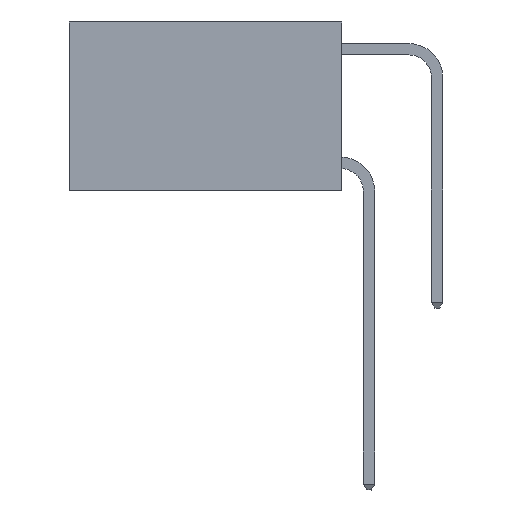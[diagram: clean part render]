
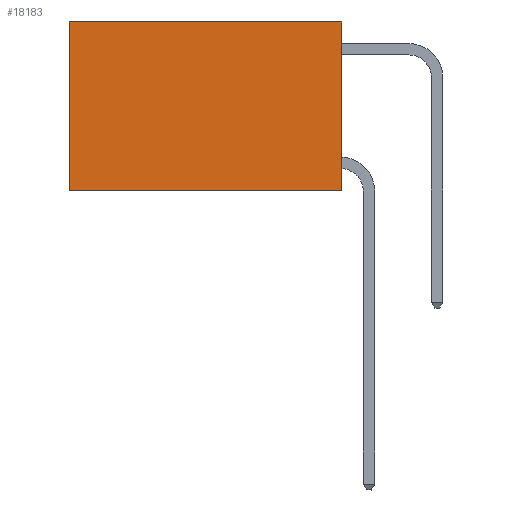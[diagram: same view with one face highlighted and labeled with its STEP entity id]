
A CAD part, left-side view. The second image highlights one B-rep face of the part: STEP entity #18183.
In plain terms, the highlighted planar face has unit normal (-1, 0, 0).
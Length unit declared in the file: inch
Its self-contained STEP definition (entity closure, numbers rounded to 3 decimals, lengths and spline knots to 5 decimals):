
#637 = CARTESIAN_POINT ( 'NONE',  ( 0.2625, 0., 0. ) ) ;
#885 = CARTESIAN_POINT ( 'NONE',  ( 0.2625, 0., 0. ) ) ;
#1502 = VECTOR ( 'NONE', #6927, 39.37008 ) ;
#2022 = ORIENTED_EDGE ( 'NONE', *, *, #14212, .T. ) ;
#3116 = CARTESIAN_POINT ( 'NONE',  ( 0.2625, 0., -0.37 ) ) ;
#3586 = ORIENTED_EDGE ( 'NONE', *, *, #18793, .F. ) ;
#3633 = DIRECTION ( 'NONE',  ( 0., 0., -1. ) ) ;
#3837 = DIRECTION ( 'NONE',  ( 1., 0., 0. ) ) ;
#4328 = LINE ( 'NONE', #637, #23978 ) ;
#4943 = EDGE_CURVE ( 'NONE', #7924, #12172, #4328, .T. ) ;
#5233 = CARTESIAN_POINT ( 'NONE',  ( 0.2625, 0., -0.37 ) ) ;
#5463 = LINE ( 'NONE', #7539, #13343 ) ;
#5824 = CARTESIAN_POINT ( 'NONE',  ( 0.2625, 0.6, -0.37 ) ) ;
#6341 = VERTEX_POINT ( 'NONE', #5233 ) ;
#6412 = LINE ( 'NONE', #885, #7974 ) ;
#6744 = ORIENTED_EDGE ( 'NONE', *, *, #4943, .T. ) ;
#6927 = DIRECTION ( 'NONE',  ( 0., 1., 0. ) ) ;
#7294 = DIRECTION ( 'NONE',  ( 0., 0., -1. ) ) ;
#7539 = CARTESIAN_POINT ( 'NONE',  ( 0.2625, 0.6, 0. ) ) ;
#7754 = PLANE ( 'NONE',  #24263 ) ;
#7924 = VERTEX_POINT ( 'NONE', #25789 ) ;
#7974 = VECTOR ( 'NONE', #7294, 39.37008 ) ;
#8041 = EDGE_LOOP ( 'NONE', ( #2022, #8569, #3586, #6744 ) ) ;
#8569 = ORIENTED_EDGE ( 'NONE', *, *, #9414, .F. ) ;
#8909 = CARTESIAN_POINT ( 'NONE',  ( 0.2625, 0.6, 0. ) ) ;
#9414 = EDGE_CURVE ( 'NONE', #6341, #10053, #18636, .T. ) ;
#9850 = DIRECTION ( 'NONE',  ( 0., 0., -1. ) ) ;
#10053 = VERTEX_POINT ( 'NONE', #5824 ) ;
#10470 = DIRECTION ( 'NONE',  ( 0., 1., 0. ) ) ;
#12172 = VERTEX_POINT ( 'NONE', #8909 ) ;
#13343 = VECTOR ( 'NONE', #3633, 39.37008 ) ;
#14212 = EDGE_CURVE ( 'NONE', #12172, #10053, #5463, .T. ) ;
#18183 = ADVANCED_FACE ( 'NONE', ( #25694 ), #7754, .F. ) ;
#18636 = LINE ( 'NONE', #3116, #1502 ) ;
#18793 = EDGE_CURVE ( 'NONE', #7924, #6341, #6412, .T. ) ;
#21805 = CARTESIAN_POINT ( 'NONE',  ( 0.2625, 0., 0. ) ) ;
#23978 = VECTOR ( 'NONE', #10470, 39.37008 ) ;
#24263 = AXIS2_PLACEMENT_3D ( 'NONE', #21805, #3837, #9850 ) ;
#25694 = FACE_OUTER_BOUND ( 'NONE', #8041, .T. ) ;
#25789 = CARTESIAN_POINT ( 'NONE',  ( 0.2625, 0., 0. ) ) ;
